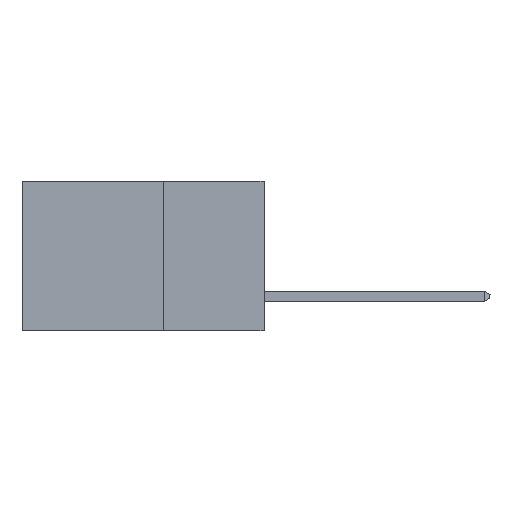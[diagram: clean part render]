
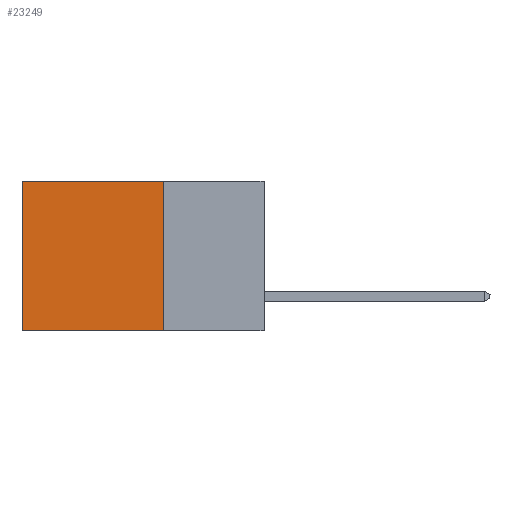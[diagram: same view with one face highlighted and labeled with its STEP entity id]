
A CAD part, left-side view. The second image highlights one B-rep face of the part: STEP entity #23249.
In plain terms, the highlighted planar face has unit normal (-1, 0, 0).
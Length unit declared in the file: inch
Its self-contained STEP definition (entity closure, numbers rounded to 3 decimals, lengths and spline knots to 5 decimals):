
#90 = VERTEX_POINT ( 'NONE', #143 ) ;
#143 = CARTESIAN_POINT ( 'NONE',  ( 0.298, 0.6, 0. ) ) ;
#1192 = EDGE_CURVE ( 'NONE', #90, #1592, #23296, .T. ) ;
#1592 = VERTEX_POINT ( 'NONE', #17226 ) ;
#1760 = CARTESIAN_POINT ( 'NONE',  ( 0.298, 0.25, -0.37 ) ) ;
#2605 = DIRECTION ( 'NONE',  ( 1., 0., 0. ) ) ;
#3373 = AXIS2_PLACEMENT_3D ( 'NONE', #13897, #2605, #19895 ) ;
#4096 = FACE_OUTER_BOUND ( 'NONE', #11947, .T. ) ;
#4928 = LINE ( 'NONE', #11335, #14356 ) ;
#5595 = DIRECTION ( 'NONE',  ( 0., 0., -1. ) ) ;
#9289 = CARTESIAN_POINT ( 'NONE',  ( 0.298, 0.25, 0. ) ) ;
#9683 = VECTOR ( 'NONE', #5595, 39.37008 ) ;
#9713 = LINE ( 'NONE', #9289, #9683 ) ;
#9956 = ORIENTED_EDGE ( 'NONE', *, *, #14549, .T. ) ;
#10380 = ORIENTED_EDGE ( 'NONE', *, *, #22484, .F. ) ;
#10765 = ORIENTED_EDGE ( 'NONE', *, *, #18181, .F. ) ;
#11335 = CARTESIAN_POINT ( 'NONE',  ( 0.298, 0.25, 0. ) ) ;
#11947 = EDGE_LOOP ( 'NONE', ( #15670, #10765, #10380, #9956 ) ) ;
#12167 = PLANE ( 'NONE',  #3373 ) ;
#13897 = CARTESIAN_POINT ( 'NONE',  ( 0.298, 0.25, 0. ) ) ;
#14102 = DIRECTION ( 'NONE',  ( 0., 0., -1. ) ) ;
#14346 = VERTEX_POINT ( 'NONE', #16856 ) ;
#14356 = VECTOR ( 'NONE', #20798, 39.37008 ) ;
#14549 = EDGE_CURVE ( 'NONE', #16358, #90, #4928, .T. ) ;
#15364 = LINE ( 'NONE', #1760, #21822 ) ;
#15670 = ORIENTED_EDGE ( 'NONE', *, *, #1192, .T. ) ;
#16358 = VERTEX_POINT ( 'NONE', #21742 ) ;
#16856 = CARTESIAN_POINT ( 'NONE',  ( 0.298, 0.25, -0.37 ) ) ;
#17226 = CARTESIAN_POINT ( 'NONE',  ( 0.298, 0.6, -0.37 ) ) ;
#18001 = VECTOR ( 'NONE', #14102, 39.37008 ) ;
#18181 = EDGE_CURVE ( 'NONE', #14346, #1592, #15364, .T. ) ;
#18875 = DIRECTION ( 'NONE',  ( 0., 1., 0. ) ) ;
#19895 = DIRECTION ( 'NONE',  ( 0., 0., -1. ) ) ;
#20798 = DIRECTION ( 'NONE',  ( 0., 1., 0. ) ) ;
#21742 = CARTESIAN_POINT ( 'NONE',  ( 0.298, 0.25, 0. ) ) ;
#21822 = VECTOR ( 'NONE', #18875, 39.37008 ) ;
#22484 = EDGE_CURVE ( 'NONE', #16358, #14346, #9713, .T. ) ;
#23249 = ADVANCED_FACE ( 'NONE', ( #4096 ), #12167, .F. ) ;
#23296 = LINE ( 'NONE', #23811, #18001 ) ;
#23811 = CARTESIAN_POINT ( 'NONE',  ( 0.298, 0.6, 0. ) ) ;
